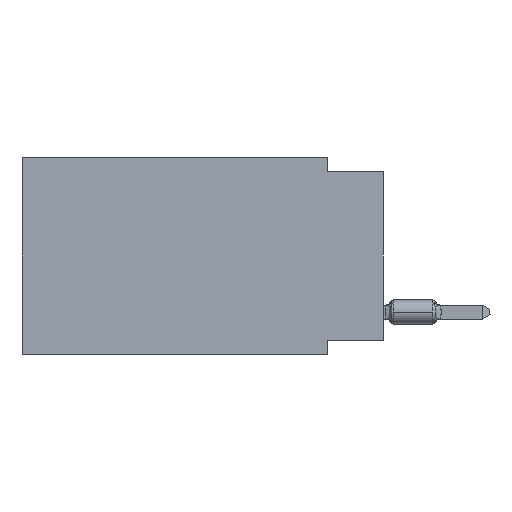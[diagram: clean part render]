
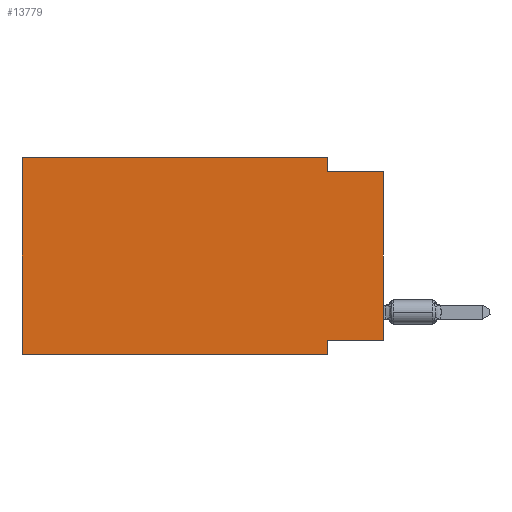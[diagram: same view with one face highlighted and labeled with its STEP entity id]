
A CAD part, left-side view. The second image highlights one B-rep face of the part: STEP entity #13779.
In plain terms, the highlighted planar face has unit normal (-1, 0, 0).
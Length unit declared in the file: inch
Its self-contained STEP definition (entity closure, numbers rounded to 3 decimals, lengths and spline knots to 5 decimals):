
#711 = LINE ( 'NONE', #67224, #58808 ) ;
#988 = CARTESIAN_POINT ( 'NONE',  ( 0., 0.1, -0.325 ) ) ;
#1951 = CARTESIAN_POINT ( 'NONE',  ( 0., 0., 0. ) ) ;
#4340 = VERTEX_POINT ( 'NONE', #22509 ) ;
#4919 = EDGE_CURVE ( 'NONE', #4340, #5828, #64003, .T. ) ;
#5828 = VERTEX_POINT ( 'NONE', #52506 ) ;
#5992 = PLANE ( 'NONE',  #46661 ) ;
#6468 = EDGE_CURVE ( 'NONE', #60084, #13174, #44972, .T. ) ;
#7642 = EDGE_LOOP ( 'NONE', ( #13233, #42678, #33428, #52833, #8453, #25696, #14090, #58377 ) ) ;
#8101 = DIRECTION ( 'NONE',  ( 0., -1., 0. ) ) ;
#8332 = LINE ( 'NONE', #57709, #67212 ) ;
#8453 = ORIENTED_EDGE ( 'NONE', *, *, #6468, .F. ) ;
#8807 = VERTEX_POINT ( 'NONE', #62281 ) ;
#9105 = CARTESIAN_POINT ( 'NONE',  ( 0., 0.645, 0. ) ) ;
#12924 = LINE ( 'NONE', #1951, #30977 ) ;
#13174 = VERTEX_POINT ( 'NONE', #27036 ) ;
#13233 = ORIENTED_EDGE ( 'NONE', *, *, #43014, .T. ) ;
#13627 = DIRECTION ( 'NONE',  ( 0., 0., -1. ) ) ;
#13779 = ADVANCED_FACE ( 'NONE', ( #56074 ), #5992, .F. ) ;
#14090 = ORIENTED_EDGE ( 'NONE', *, *, #44090, .F. ) ;
#14734 = EDGE_CURVE ( 'NONE', #8807, #66444, #14893, .T. ) ;
#14893 = LINE ( 'NONE', #66026, #22304 ) ;
#20718 = LINE ( 'NONE', #21812, #53631 ) ;
#21812 = CARTESIAN_POINT ( 'NONE',  ( 0., 0.1, 0. ) ) ;
#22304 = VECTOR ( 'NONE', #70778, 39.37008 ) ;
#22509 = CARTESIAN_POINT ( 'NONE',  ( 0., 0.1, -0.025 ) ) ;
#22824 = DIRECTION ( 'NONE',  ( 1., 0., 0. ) ) ;
#25614 = LINE ( 'NONE', #9105, #42386 ) ;
#25696 = ORIENTED_EDGE ( 'NONE', *, *, #31964, .T. ) ;
#26546 = EDGE_CURVE ( 'NONE', #68556, #4340, #20718, .T. ) ;
#27036 = CARTESIAN_POINT ( 'NONE',  ( 0., 0.645, 0. ) ) ;
#27038 = DIRECTION ( 'NONE',  ( 0., -1., 0. ) ) ;
#28220 = CARTESIAN_POINT ( 'NONE',  ( 0., 0.645, -0.35 ) ) ;
#28665 = DIRECTION ( 'NONE',  ( 0., 0., 1. ) ) ;
#30977 = VECTOR ( 'NONE', #28665, 39.37008 ) ;
#31964 = EDGE_CURVE ( 'NONE', #60084, #58928, #711, .T. ) ;
#33428 = ORIENTED_EDGE ( 'NONE', *, *, #26546, .F. ) ;
#35038 = DIRECTION ( 'NONE',  ( 0., 0., 1. ) ) ;
#35445 = CARTESIAN_POINT ( 'NONE',  ( 0., 0.1, -0.35 ) ) ;
#36233 = CARTESIAN_POINT ( 'NONE',  ( 0., 0., -0.025 ) ) ;
#39462 = CARTESIAN_POINT ( 'NONE',  ( 0., 0.645, 0. ) ) ;
#40552 = DIRECTION ( 'NONE',  ( 0., -1., 0. ) ) ;
#42386 = VECTOR ( 'NONE', #27038, 39.37008 ) ;
#42678 = ORIENTED_EDGE ( 'NONE', *, *, #4919, .F. ) ;
#43014 = EDGE_CURVE ( 'NONE', #8807, #5828, #12924, .T. ) ;
#43972 = CARTESIAN_POINT ( 'NONE',  ( 0., 0.1, 0. ) ) ;
#44090 = EDGE_CURVE ( 'NONE', #66444, #58928, #8332, .T. ) ;
#44972 = LINE ( 'NONE', #39462, #69824 ) ;
#46661 = AXIS2_PLACEMENT_3D ( 'NONE', #50604, #22824, #13627 ) ;
#48293 = EDGE_CURVE ( 'NONE', #13174, #68556, #25614, .T. ) ;
#50604 = CARTESIAN_POINT ( 'NONE',  ( 0., 0.645, 0. ) ) ;
#52506 = CARTESIAN_POINT ( 'NONE',  ( 0., 0., -0.025 ) ) ;
#52833 = ORIENTED_EDGE ( 'NONE', *, *, #48293, .F. ) ;
#53631 = VECTOR ( 'NONE', #65270, 39.37008 ) ;
#56074 = FACE_OUTER_BOUND ( 'NONE', #7642, .T. ) ;
#57709 = CARTESIAN_POINT ( 'NONE',  ( 0., 0.1, -0.35 ) ) ;
#58377 = ORIENTED_EDGE ( 'NONE', *, *, #14734, .F. ) ;
#58808 = VECTOR ( 'NONE', #40552, 39.37008 ) ;
#58928 = VERTEX_POINT ( 'NONE', #35445 ) ;
#60084 = VERTEX_POINT ( 'NONE', #28220 ) ;
#62281 = CARTESIAN_POINT ( 'NONE',  ( 0., 0., -0.325 ) ) ;
#64003 = LINE ( 'NONE', #36233, #69761 ) ;
#65270 = DIRECTION ( 'NONE',  ( 0., 0., -1. ) ) ;
#66026 = CARTESIAN_POINT ( 'NONE',  ( 0., 0., -0.325 ) ) ;
#66444 = VERTEX_POINT ( 'NONE', #988 ) ;
#67212 = VECTOR ( 'NONE', #69340, 39.37008 ) ;
#67224 = CARTESIAN_POINT ( 'NONE',  ( 0., 0.645, -0.35 ) ) ;
#68556 = VERTEX_POINT ( 'NONE', #43972 ) ;
#69340 = DIRECTION ( 'NONE',  ( 0., 0., -1. ) ) ;
#69761 = VECTOR ( 'NONE', #8101, 39.37008 ) ;
#69824 = VECTOR ( 'NONE', #35038, 39.37008 ) ;
#70778 = DIRECTION ( 'NONE',  ( 0., 1., 0. ) ) ;
